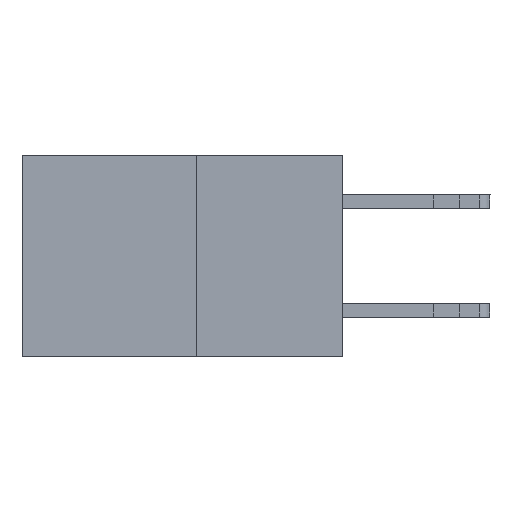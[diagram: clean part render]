
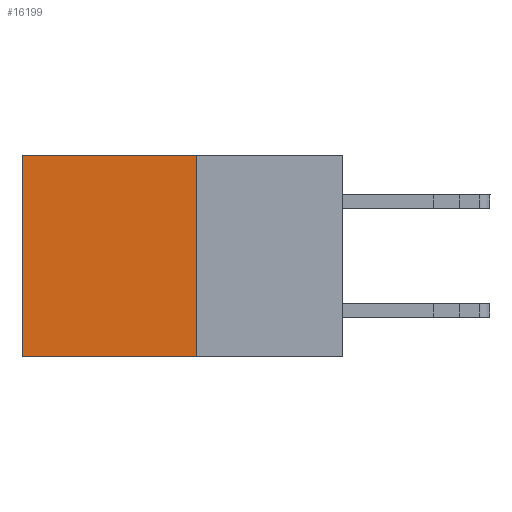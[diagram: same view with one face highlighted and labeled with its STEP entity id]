
A CAD part, left-side view. The second image highlights one B-rep face of the part: STEP entity #16199.
In plain terms, the highlighted planar face has unit normal (-1, 0, 0).
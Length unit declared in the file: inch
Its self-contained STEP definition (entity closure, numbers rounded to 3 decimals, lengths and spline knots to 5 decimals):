
#24 = PLANE ( 'NONE',  #11743 ) ;
#150 = ORIENTED_EDGE ( 'NONE', *, *, #5992, .T. ) ;
#1236 = LINE ( 'NONE', #14704, #14821 ) ;
#2765 = EDGE_CURVE ( 'NONE', #10901, #26705, #17707, .T. ) ;
#2960 = CARTESIAN_POINT ( 'NONE',  ( 0.277, 0.27, -0.37 ) ) ;
#3674 = VERTEX_POINT ( 'NONE', #26896 ) ;
#4815 = DIRECTION ( 'NONE',  ( 1., 0., 0. ) ) ;
#5992 = EDGE_CURVE ( 'NONE', #29908, #26705, #1236, .T. ) ;
#7542 = EDGE_CURVE ( 'NONE', #3674, #10901, #27425, .T. ) ;
#8228 = EDGE_LOOP ( 'NONE', ( #150, #8444, #12251, #12627 ) ) ;
#8444 = ORIENTED_EDGE ( 'NONE', *, *, #2765, .F. ) ;
#8862 = DIRECTION ( 'NONE',  ( 0., 1., 0. ) ) ;
#10901 = VERTEX_POINT ( 'NONE', #19506 ) ;
#11743 = AXIS2_PLACEMENT_3D ( 'NONE', #2960, #4815, #21435 ) ;
#11985 = FACE_OUTER_BOUND ( 'NONE', #8228, .T. ) ;
#12251 = ORIENTED_EDGE ( 'NONE', *, *, #7542, .F. ) ;
#12627 = ORIENTED_EDGE ( 'NONE', *, *, #25614, .T. ) ;
#14303 = VECTOR ( 'NONE', #8862, 39.37008 ) ;
#14501 = CARTESIAN_POINT ( 'NONE',  ( 0.277, 0.27, 0. ) ) ;
#14704 = CARTESIAN_POINT ( 'NONE',  ( 0.277, 0.59, -0.37 ) ) ;
#14821 = VECTOR ( 'NONE', #20145, 39.37008 ) ;
#16199 = ADVANCED_FACE ( 'NONE', ( #11985 ), #24, .F. ) ;
#17707 = LINE ( 'NONE', #17860, #14303 ) ;
#17860 = CARTESIAN_POINT ( 'NONE',  ( 0.277, 0.27, -0.37 ) ) ;
#19506 = CARTESIAN_POINT ( 'NONE',  ( 0.277, 0.27, -0.37 ) ) ;
#20145 = DIRECTION ( 'NONE',  ( 0., 0., -1. ) ) ;
#20386 = CARTESIAN_POINT ( 'NONE',  ( 0.277, 0.59, 0. ) ) ;
#20936 = VECTOR ( 'NONE', #25967, 39.37008 ) ;
#21435 = DIRECTION ( 'NONE',  ( 0., 0., -1. ) ) ;
#24798 = CARTESIAN_POINT ( 'NONE',  ( 0.277, 0.27, -0.37 ) ) ;
#25102 = DIRECTION ( 'NONE',  ( 0., 0., -1. ) ) ;
#25237 = VECTOR ( 'NONE', #25102, 39.37008 ) ;
#25614 = EDGE_CURVE ( 'NONE', #3674, #29908, #25813, .T. ) ;
#25813 = LINE ( 'NONE', #14501, #20936 ) ;
#25967 = DIRECTION ( 'NONE',  ( 0., 1., 0. ) ) ;
#26705 = VERTEX_POINT ( 'NONE', #29138 ) ;
#26896 = CARTESIAN_POINT ( 'NONE',  ( 0.277, 0.27, 0. ) ) ;
#27425 = LINE ( 'NONE', #24798, #25237 ) ;
#29138 = CARTESIAN_POINT ( 'NONE',  ( 0.277, 0.59, -0.37 ) ) ;
#29908 = VERTEX_POINT ( 'NONE', #20386 ) ;
